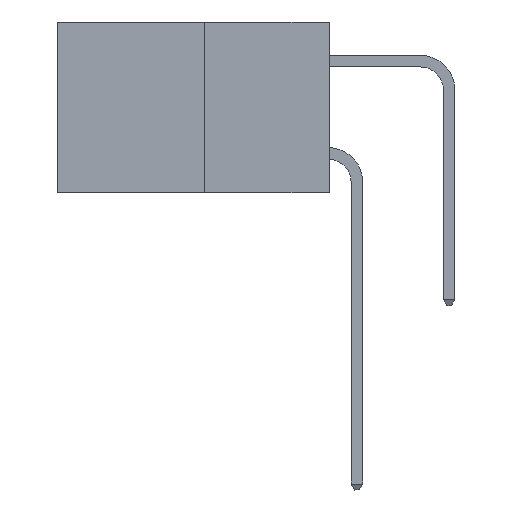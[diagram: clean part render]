
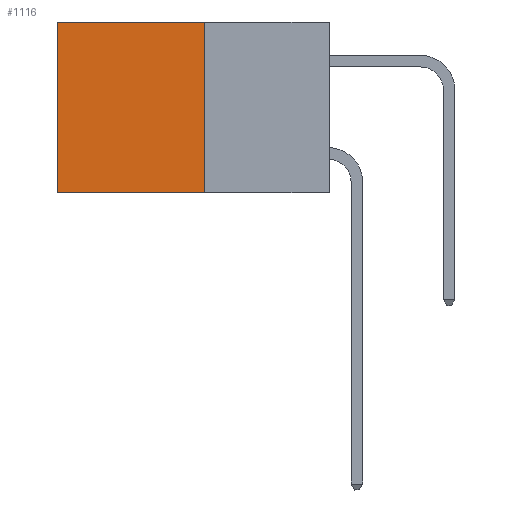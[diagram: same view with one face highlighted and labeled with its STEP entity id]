
A CAD part, left-side view. The second image highlights one B-rep face of the part: STEP entity #1116.
In plain terms, the highlighted planar face has unit normal (-1, 0, 0).
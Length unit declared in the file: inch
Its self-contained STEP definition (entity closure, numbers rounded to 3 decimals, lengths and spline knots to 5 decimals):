
#693 = EDGE_CURVE ( 'NONE', #9959, #5440, #8288, .T. ) ;
#1116 = ADVANCED_FACE ( 'NONE', ( #8386 ), #6535, .F. ) ;
#1144 = DIRECTION ( 'NONE',  ( 0., 0., -1. ) ) ;
#1290 = DIRECTION ( 'NONE',  ( 0., 1., 0. ) ) ;
#1513 = EDGE_LOOP ( 'NONE', ( #8780, #5987, #5037, #3357 ) ) ;
#1550 = CARTESIAN_POINT ( 'NONE',  ( 0.277, 0.27, -0.37 ) ) ;
#2127 = CARTESIAN_POINT ( 'NONE',  ( 0.277, 0.27, 0. ) ) ;
#3053 = VECTOR ( 'NONE', #1144, 39.37008 ) ;
#3066 = DIRECTION ( 'NONE',  ( 0., 1., 0. ) ) ;
#3273 = EDGE_CURVE ( 'NONE', #7157, #5725, #6698, .T. ) ;
#3314 = LINE ( 'NONE', #5471, #3053 ) ;
#3357 = ORIENTED_EDGE ( 'NONE', *, *, #3273, .T. ) ;
#3639 = VECTOR ( 'NONE', #8956, 39.37008 ) ;
#3979 = EDGE_CURVE ( 'NONE', #7157, #9959, #3314, .T. ) ;
#5037 = ORIENTED_EDGE ( 'NONE', *, *, #3979, .F. ) ;
#5440 = VERTEX_POINT ( 'NONE', #9168 ) ;
#5441 = CARTESIAN_POINT ( 'NONE',  ( 0.277, 0.27, -0.37 ) ) ;
#5471 = CARTESIAN_POINT ( 'NONE',  ( 0.277, 0.27, -0.37 ) ) ;
#5725 = VERTEX_POINT ( 'NONE', #9387 ) ;
#5938 = CARTESIAN_POINT ( 'NONE',  ( 0.277, 0.27, 0. ) ) ;
#5978 = VECTOR ( 'NONE', #1290, 39.37008 ) ;
#5987 = ORIENTED_EDGE ( 'NONE', *, *, #693, .F. ) ;
#6135 = EDGE_CURVE ( 'NONE', #5725, #5440, #9938, .T. ) ;
#6487 = CARTESIAN_POINT ( 'NONE',  ( 0.277, 0.27, -0.37 ) ) ;
#6535 = PLANE ( 'NONE',  #9203 ) ;
#6698 = LINE ( 'NONE', #2127, #8746 ) ;
#6713 = DIRECTION ( 'NONE',  ( 0., 0., -1. ) ) ;
#7157 = VERTEX_POINT ( 'NONE', #5938 ) ;
#7392 = CARTESIAN_POINT ( 'NONE',  ( 0.277, 0.59, -0.37 ) ) ;
#8288 = LINE ( 'NONE', #1550, #5978 ) ;
#8386 = FACE_OUTER_BOUND ( 'NONE', #1513, .T. ) ;
#8746 = VECTOR ( 'NONE', #3066, 39.37008 ) ;
#8780 = ORIENTED_EDGE ( 'NONE', *, *, #6135, .T. ) ;
#8921 = DIRECTION ( 'NONE',  ( 1., 0., 0. ) ) ;
#8956 = DIRECTION ( 'NONE',  ( 0., 0., -1. ) ) ;
#9168 = CARTESIAN_POINT ( 'NONE',  ( 0.277, 0.59, -0.37 ) ) ;
#9203 = AXIS2_PLACEMENT_3D ( 'NONE', #6487, #8921, #6713 ) ;
#9387 = CARTESIAN_POINT ( 'NONE',  ( 0.277, 0.59, 0. ) ) ;
#9938 = LINE ( 'NONE', #7392, #3639 ) ;
#9959 = VERTEX_POINT ( 'NONE', #5441 ) ;
